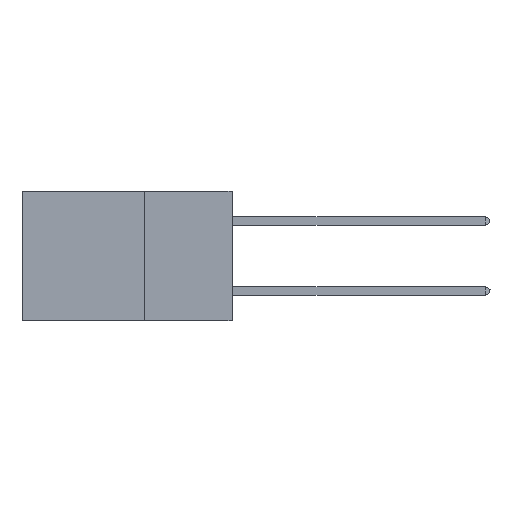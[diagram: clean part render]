
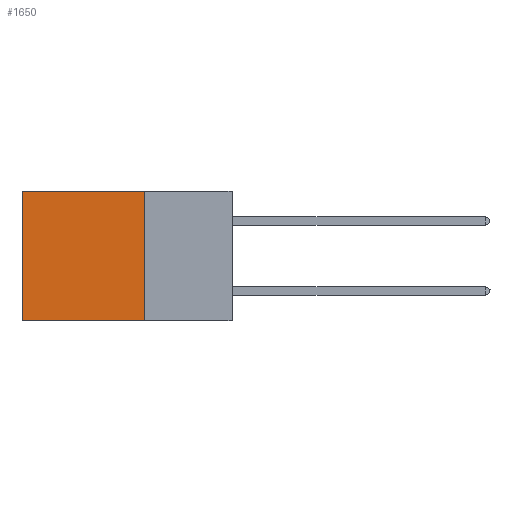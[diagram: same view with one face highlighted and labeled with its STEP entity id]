
A CAD part, left-side view. The second image highlights one B-rep face of the part: STEP entity #1650.
In plain terms, the highlighted planar face has unit normal (-1, 0, 0).
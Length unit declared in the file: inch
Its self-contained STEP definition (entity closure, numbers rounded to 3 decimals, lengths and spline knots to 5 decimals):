
#222 = VECTOR ( 'NONE', #3829, 39.37008 ) ;
#1650 = ADVANCED_FACE ( 'NONE', ( #4237 ), #20549, .F. ) ;
#2305 = EDGE_LOOP ( 'NONE', ( #30099, #4207, #27497, #11602 ) ) ;
#2947 = CARTESIAN_POINT ( 'NONE',  ( 0.2875, 0.25, -0.37 ) ) ;
#3366 = VERTEX_POINT ( 'NONE', #10209 ) ;
#3829 = DIRECTION ( 'NONE',  ( 0., 0., -1. ) ) ;
#4207 = ORIENTED_EDGE ( 'NONE', *, *, #20441, .F. ) ;
#4237 = FACE_OUTER_BOUND ( 'NONE', #2305, .T. ) ;
#5037 = CARTESIAN_POINT ( 'NONE',  ( 0.2875, 0.25, 0. ) ) ;
#9114 = DIRECTION ( 'NONE',  ( 0., 0., -1. ) ) ;
#9830 = EDGE_CURVE ( 'NONE', #19672, #13515, #32677, .T. ) ;
#10209 = CARTESIAN_POINT ( 'NONE',  ( 0.2875, 0.25, -0.37 ) ) ;
#11586 = VERTEX_POINT ( 'NONE', #32304 ) ;
#11602 = ORIENTED_EDGE ( 'NONE', *, *, #9830, .T. ) ;
#12159 = DIRECTION ( 'NONE',  ( 0., 0., -1. ) ) ;
#12946 = DIRECTION ( 'NONE',  ( 0., 1., 0. ) ) ;
#13515 = VERTEX_POINT ( 'NONE', #38012 ) ;
#16523 = VECTOR ( 'NONE', #9114, 39.37008 ) ;
#17388 = LINE ( 'NONE', #32182, #222 ) ;
#19289 = EDGE_CURVE ( 'NONE', #13515, #11586, #34375, .T. ) ;
#19672 = VERTEX_POINT ( 'NONE', #39721 ) ;
#20441 = EDGE_CURVE ( 'NONE', #3366, #11586, #28759, .T. ) ;
#20549 = PLANE ( 'NONE',  #36749 ) ;
#22433 = DIRECTION ( 'NONE',  ( 0., 1., 0. ) ) ;
#25358 = CARTESIAN_POINT ( 'NONE',  ( 0.2875, 0.25, 0. ) ) ;
#27441 = DIRECTION ( 'NONE',  ( 1., 0., 0. ) ) ;
#27497 = ORIENTED_EDGE ( 'NONE', *, *, #34438, .F. ) ;
#28759 = LINE ( 'NONE', #2947, #32236 ) ;
#30099 = ORIENTED_EDGE ( 'NONE', *, *, #19289, .T. ) ;
#31333 = CARTESIAN_POINT ( 'NONE',  ( 0.2875, 0.6, 0. ) ) ;
#32182 = CARTESIAN_POINT ( 'NONE',  ( 0.2875, 0.25, 0. ) ) ;
#32236 = VECTOR ( 'NONE', #12946, 39.37008 ) ;
#32304 = CARTESIAN_POINT ( 'NONE',  ( 0.2875, 0.6, -0.37 ) ) ;
#32677 = LINE ( 'NONE', #25358, #37603 ) ;
#34375 = LINE ( 'NONE', #31333, #16523 ) ;
#34438 = EDGE_CURVE ( 'NONE', #19672, #3366, #17388, .T. ) ;
#36749 = AXIS2_PLACEMENT_3D ( 'NONE', #5037, #27441, #12159 ) ;
#37603 = VECTOR ( 'NONE', #22433, 39.37008 ) ;
#38012 = CARTESIAN_POINT ( 'NONE',  ( 0.2875, 0.6, 0. ) ) ;
#39721 = CARTESIAN_POINT ( 'NONE',  ( 0.2875, 0.25, 0. ) ) ;
